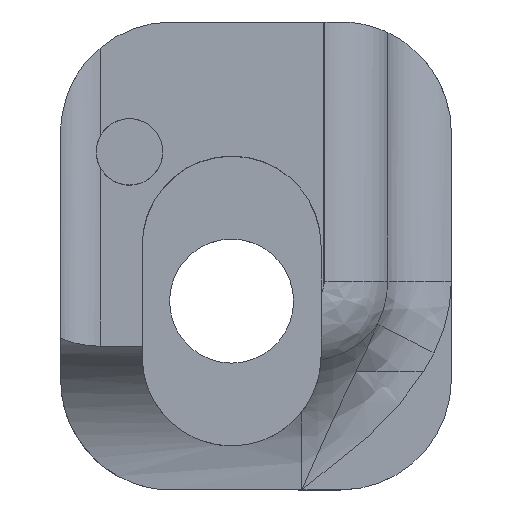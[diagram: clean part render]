
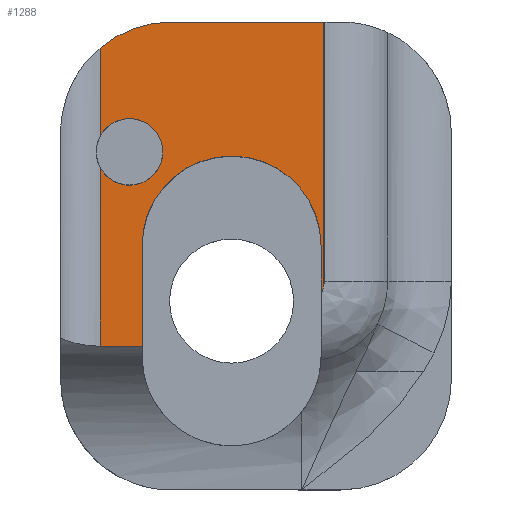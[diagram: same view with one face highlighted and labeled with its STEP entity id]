
A CAD part, top view. The second image highlights one B-rep face of the part: STEP entity #1288.
In plain terms, the highlighted planar face has unit normal (0, 0, 1).
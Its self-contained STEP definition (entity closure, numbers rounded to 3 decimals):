
#13 = VERTEX_POINT ( 'NONE', #1091 ) ;
#50 = ORIENTED_EDGE ( 'NONE', *, *, #758, .T. ) ;
#54 = CARTESIAN_POINT ( 'NONE',  ( 61.194, 16.497, 48.265 ) ) ;
#72 = ORIENTED_EDGE ( 'NONE', *, *, #1254, .F. ) ;
#93 = DIRECTION ( 'NONE',  ( 0., 0., -1. ) ) ;
#109 = EDGE_CURVE ( 'NONE', #13, #177, #979, .T. ) ;
#119 = VECTOR ( 'NONE', #926, 1000. ) ;
#127 = AXIS2_PLACEMENT_3D ( 'NONE', #961, #93, #1575 ) ;
#128 = ORIENTED_EDGE ( 'NONE', *, *, #1466, .F. ) ;
#151 = CARTESIAN_POINT ( 'NONE',  ( 61.148, 18.606, 48.265 ) ) ;
#177 = VERTEX_POINT ( 'NONE', #976 ) ;
#191 = AXIS2_PLACEMENT_3D ( 'NONE', #364, #1236, #496 ) ;
#195 = CARTESIAN_POINT ( 'NONE',  ( 53.071, 14.061, 48.265 ) ) ;
#209 = ORIENTED_EDGE ( 'NONE', *, *, #1307, .F. ) ;
#218 = EDGE_CURVE ( 'NONE', #1298, #1531, #906, .T. ) ;
#227 = DIRECTION ( 'NONE',  ( 0., 0., 1. ) ) ;
#244 = ORIENTED_EDGE ( 'NONE', *, *, #287, .T. ) ;
#258 = EDGE_CURVE ( 'NONE', #959, #936, #1056, .T. ) ;
#287 = EDGE_CURVE ( 'NONE', #436, #1446, #401, .T. ) ;
#288 = VERTEX_POINT ( 'NONE', #1380 ) ;
#293 = CARTESIAN_POINT ( 'NONE',  ( 61.275, 16.829, 48.265 ) ) ;
#312 = VECTOR ( 'NONE', #1474, 1000. ) ;
#334 = ORIENTED_EDGE ( 'NONE', *, *, #568, .F. ) ;
#364 = CARTESIAN_POINT ( 'NONE',  ( 54.391, 23.696, 48.265 ) ) ;
#365 = CARTESIAN_POINT ( 'NONE',  ( 53.071, 18.606, 48.265 ) ) ;
#397 = CARTESIAN_POINT ( 'NONE',  ( 135.443, 1.817, 48.265 ) ) ;
#401 = CIRCLE ( 'NONE', #127, 1.5 ) ;
#403 = EDGE_LOOP ( 'NONE', ( #1438, #1493, #1037, #50, #244, #1176, #1479, #334, #128, #1392, #209, #72 ) ) ;
#407 = EDGE_CURVE ( 'NONE', #509, #1400, #617, .T. ) ;
#417 = LINE ( 'NONE', #563, #119 ) ;
#436 = VERTEX_POINT ( 'NONE', #1230 ) ;
#474 = CARTESIAN_POINT ( 'NONE',  ( 51.172, 22.136, 48.265 ) ) ;
#484 = DIRECTION ( 'NONE',  ( 0., 1., 0. ) ) ;
#486 = CARTESIAN_POINT ( 'NONE',  ( 51.172, 27.521, 48.265 ) ) ;
#496 = DIRECTION ( 'NONE',  ( 1., 0., 0. ) ) ;
#509 = VERTEX_POINT ( 'NONE', #195 ) ;
#543 = AXIS2_PLACEMENT_3D ( 'NONE', #397, #1383, #651 ) ;
#563 = CARTESIAN_POINT ( 'NONE',  ( 53.071, 1.817, 48.265 ) ) ;
#568 = EDGE_CURVE ( 'NONE', #753, #509, #417, .T. ) ;
#593 = CARTESIAN_POINT ( 'NONE',  ( 51.172, 14.061, 48.265 ) ) ;
#617 = LINE ( 'NONE', #1241, #1547 ) ;
#623 = CARTESIAN_POINT ( 'NONE',  ( 135.443, 28.696, 48.265 ) ) ;
#624 = DIRECTION ( 'NONE',  ( -1., 0., 0. ) ) ;
#632 = CARTESIAN_POINT ( 'NONE',  ( 51.172, 26.175, 48.265 ) ) ;
#639 = LINE ( 'NONE', #1603, #1573 ) ;
#651 = DIRECTION ( 'NONE',  ( 1., 0., 0. ) ) ;
#672 = CIRCLE ( 'NONE', #191, 5. ) ;
#728 = VECTOR ( 'NONE', #1498, 1000. ) ;
#745 = DIRECTION ( 'NONE',  ( 0., 0., -1. ) ) ;
#753 = VERTEX_POINT ( 'NONE', #365 ) ;
#758 = EDGE_CURVE ( 'NONE', #1298, #436, #1203, .T. ) ;
#790 = CARTESIAN_POINT ( 'NONE',  ( 51.172, 23.523, 48.265 ) ) ;
#794 = CARTESIAN_POINT ( 'NONE',  ( 61.228, 16.596, 48.265 ) ) ;
#877 = B_SPLINE_CURVE_WITH_KNOTS ( 'NONE', 3,
 ( #293, #1284, #1529, #794, #54, #916 ),
 .UNSPECIFIED., .F., .F.,
 ( 4, 2, 4 ),
 ( 0., 0., 0.001 ),
 .UNSPECIFIED. ) ;
#890 = CARTESIAN_POINT ( 'NONE',  ( 61.148, 1.817, 48.265 ) ) ;
#902 = CARTESIAN_POINT ( 'NONE',  ( 61.148, 16.404, 48.265 ) ) ;
#906 = LINE ( 'NONE', #632, #1231 ) ;
#916 = CARTESIAN_POINT ( 'NONE',  ( 61.148, 16.404, 48.265 ) ) ;
#926 = DIRECTION ( 'NONE',  ( 0., -1., 0. ) ) ;
#930 = AXIS2_PLACEMENT_3D ( 'NONE', #1480, #745, #1604 ) ;
#936 = VERTEX_POINT ( 'NONE', #151 ) ;
#959 = VERTEX_POINT ( 'NONE', #902 ) ;
#961 = CARTESIAN_POINT ( 'NONE',  ( 52.502, 22.829, 48.265 ) ) ;
#970 = CARTESIAN_POINT ( 'NONE',  ( 57.11, 18.606, 48.265 ) ) ;
#976 = CARTESIAN_POINT ( 'NONE',  ( 61.274, 28.696, 48.265 ) ) ;
#979 = LINE ( 'NONE', #623, #312 ) ;
#983 = EDGE_CURVE ( 'NONE', #1400, #1446, #1339, .T. ) ;
#1035 = CARTESIAN_POINT ( 'NONE',  ( 51.172, 26.175, 48.265 ) ) ;
#1037 = ORIENTED_EDGE ( 'NONE', *, *, #218, .F. ) ;
#1055 = VECTOR ( 'NONE', #1150, 1000. ) ;
#1056 = LINE ( 'NONE', #890, #728 ) ;
#1091 = CARTESIAN_POINT ( 'NONE',  ( 54.391, 28.696, 48.265 ) ) ;
#1098 = DIRECTION ( 'NONE',  ( 1., 0., 0. ) ) ;
#1125 = AXIS2_PLACEMENT_3D ( 'NONE', #970, #227, #1098 ) ;
#1150 = DIRECTION ( 'NONE',  ( 0., 1., 0. ) ) ;
#1176 = ORIENTED_EDGE ( 'NONE', *, *, #983, .F. ) ;
#1184 = EDGE_CURVE ( 'NONE', #13, #1531, #672, .T. ) ;
#1203 = CIRCLE ( 'NONE', #930, 1.5 ) ;
#1230 = CARTESIAN_POINT ( 'NONE',  ( 54.002, 22.829, 48.265 ) ) ;
#1231 = VECTOR ( 'NONE', #484, 1000. ) ;
#1236 = DIRECTION ( 'NONE',  ( 0., 0., 1. ) ) ;
#1241 = CARTESIAN_POINT ( 'NONE',  ( 75.363, 14.061, 48.265 ) ) ;
#1245 = DIRECTION ( 'NONE',  ( 0., -1., 0. ) ) ;
#1253 = FACE_OUTER_BOUND ( 'NONE', #403, .T. ) ;
#1254 = EDGE_CURVE ( 'NONE', #177, #288, #639, .T. ) ;
#1260 = PLANE ( 'NONE',  #543 ) ;
#1284 = CARTESIAN_POINT ( 'NONE',  ( 61.269, 16.784, 48.265 ) ) ;
#1288 = ADVANCED_FACE ( 'NONE', ( #1253 ), #1260, .F. ) ;
#1298 = VERTEX_POINT ( 'NONE', #790 ) ;
#1307 = EDGE_CURVE ( 'NONE', #288, #959, #877, .T. ) ;
#1339 = LINE ( 'NONE', #1035, #1055 ) ;
#1380 = CARTESIAN_POINT ( 'NONE',  ( 61.275, 16.829, 48.265 ) ) ;
#1383 = DIRECTION ( 'NONE',  ( 0., 0., -1. ) ) ;
#1392 = ORIENTED_EDGE ( 'NONE', *, *, #258, .F. ) ;
#1400 = VERTEX_POINT ( 'NONE', #593 ) ;
#1418 = CIRCLE ( 'NONE', #1125, 4.039 ) ;
#1438 = ORIENTED_EDGE ( 'NONE', *, *, #109, .F. ) ;
#1446 = VERTEX_POINT ( 'NONE', #474 ) ;
#1466 = EDGE_CURVE ( 'NONE', #936, #753, #1418, .T. ) ;
#1474 = DIRECTION ( 'NONE',  ( 1., 0., 0. ) ) ;
#1479 = ORIENTED_EDGE ( 'NONE', *, *, #407, .F. ) ;
#1480 = CARTESIAN_POINT ( 'NONE',  ( 52.502, 22.829, 48.265 ) ) ;
#1493 = ORIENTED_EDGE ( 'NONE', *, *, #1184, .T. ) ;
#1498 = DIRECTION ( 'NONE',  ( 0., 1., 0. ) ) ;
#1529 = CARTESIAN_POINT ( 'NONE',  ( 61.261, 16.74, 48.265 ) ) ;
#1531 = VERTEX_POINT ( 'NONE', #486 ) ;
#1547 = VECTOR ( 'NONE', #624, 1000. ) ;
#1573 = VECTOR ( 'NONE', #1245, 1000. ) ;
#1575 = DIRECTION ( 'NONE',  ( 1., 0., 0. ) ) ;
#1603 = CARTESIAN_POINT ( 'NONE',  ( 61.274, 17.001, 48.265 ) ) ;
#1604 = DIRECTION ( 'NONE',  ( 1., 0., 0. ) ) ;
